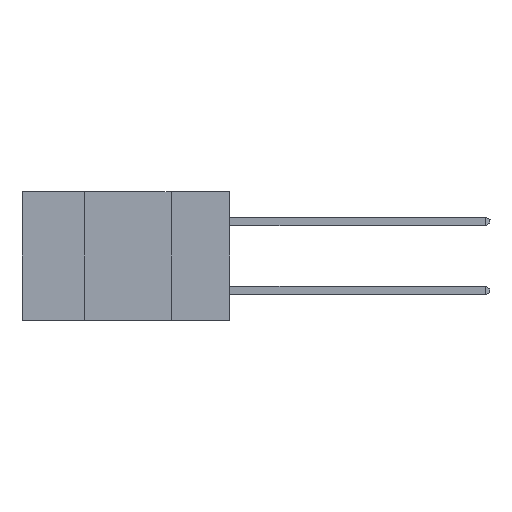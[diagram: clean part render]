
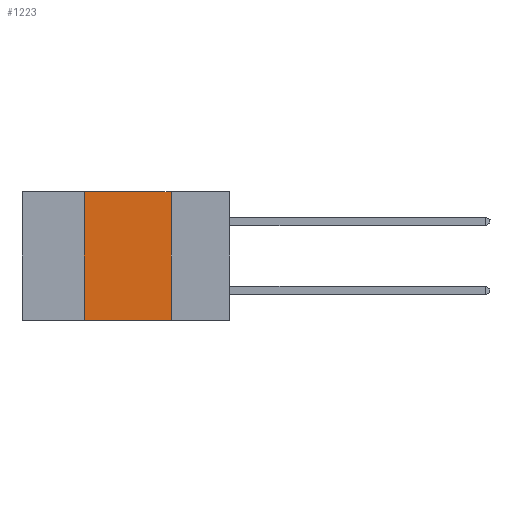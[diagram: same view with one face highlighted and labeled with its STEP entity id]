
A CAD part, left-side view. The second image highlights one B-rep face of the part: STEP entity #1223.
In plain terms, the highlighted planar face has unit normal (-1, 0, 0).
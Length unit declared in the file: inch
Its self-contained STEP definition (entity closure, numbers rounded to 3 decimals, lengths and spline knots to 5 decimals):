
#252 = EDGE_CURVE ( 'NONE', #29274, #27640, #12813, .T. ) ;
#1223 = ADVANCED_FACE ( 'NONE', ( #29236 ), #24031, .F. ) ;
#2565 = EDGE_LOOP ( 'NONE', ( #30117, #15206, #2757, #25941 ) ) ;
#2757 = ORIENTED_EDGE ( 'NONE', *, *, #3627, .F. ) ;
#2820 = VERTEX_POINT ( 'NONE', #3161 ) ;
#3161 = CARTESIAN_POINT ( 'NONE',  ( 0., 0.42, 0. ) ) ;
#3627 = EDGE_CURVE ( 'NONE', #29274, #2820, #13788, .T. ) ;
#6244 = VECTOR ( 'NONE', #29291, 39.37008 ) ;
#7065 = EDGE_CURVE ( 'NONE', #2820, #12545, #17566, .T. ) ;
#7499 = CARTESIAN_POINT ( 'NONE',  ( 0., 0.17, 0. ) ) ;
#12287 = CARTESIAN_POINT ( 'NONE',  ( 0., 0.6, -0.37 ) ) ;
#12545 = VERTEX_POINT ( 'NONE', #7499 ) ;
#12813 = LINE ( 'NONE', #12287, #6244 ) ;
#13013 = VECTOR ( 'NONE', #25266, 39.37008 ) ;
#13788 = LINE ( 'NONE', #25263, #13013 ) ;
#15206 = ORIENTED_EDGE ( 'NONE', *, *, #7065, .F. ) ;
#15377 = AXIS2_PLACEMENT_3D ( 'NONE', #22459, #28154, #18646 ) ;
#17566 = LINE ( 'NONE', #20090, #30527 ) ;
#18646 = DIRECTION ( 'NONE',  ( 0., 0., -1. ) ) ;
#19055 = DIRECTION ( 'NONE',  ( 0., -1., 0. ) ) ;
#19186 = EDGE_CURVE ( 'NONE', #12545, #27640, #30349, .T. ) ;
#20090 = CARTESIAN_POINT ( 'NONE',  ( 0., 0.6, 0. ) ) ;
#21229 = CARTESIAN_POINT ( 'NONE',  ( 0., 0.42, -0.37 ) ) ;
#21545 = DIRECTION ( 'NONE',  ( 0., 0., -1. ) ) ;
#22459 = CARTESIAN_POINT ( 'NONE',  ( 0., 0.6, 0. ) ) ;
#23130 = VECTOR ( 'NONE', #21545, 39.37008 ) ;
#23861 = CARTESIAN_POINT ( 'NONE',  ( 0., 0.17, 0. ) ) ;
#24031 = PLANE ( 'NONE',  #15377 ) ;
#25263 = CARTESIAN_POINT ( 'NONE',  ( 0., 0.42, 0. ) ) ;
#25266 = DIRECTION ( 'NONE',  ( 0., 0., 1. ) ) ;
#25941 = ORIENTED_EDGE ( 'NONE', *, *, #252, .T. ) ;
#27116 = CARTESIAN_POINT ( 'NONE',  ( 0., 0.17, -0.37 ) ) ;
#27640 = VERTEX_POINT ( 'NONE', #27116 ) ;
#28154 = DIRECTION ( 'NONE',  ( 1., 0., 0. ) ) ;
#29236 = FACE_OUTER_BOUND ( 'NONE', #2565, .T. ) ;
#29274 = VERTEX_POINT ( 'NONE', #21229 ) ;
#29291 = DIRECTION ( 'NONE',  ( 0., -1., 0. ) ) ;
#30117 = ORIENTED_EDGE ( 'NONE', *, *, #19186, .F. ) ;
#30349 = LINE ( 'NONE', #23861, #23130 ) ;
#30527 = VECTOR ( 'NONE', #19055, 39.37008 ) ;
